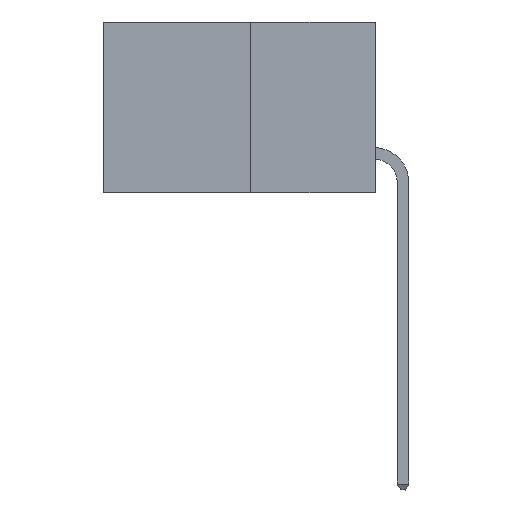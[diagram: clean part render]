
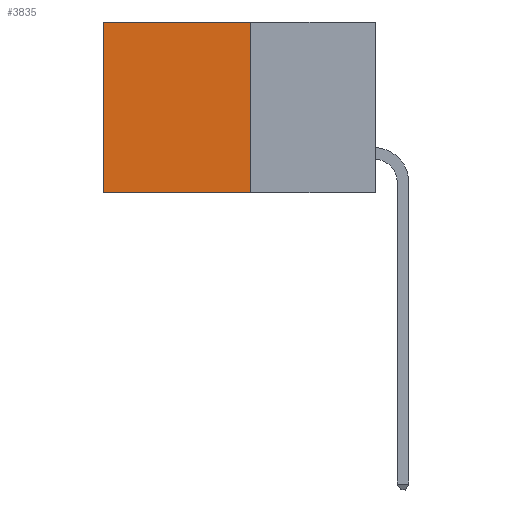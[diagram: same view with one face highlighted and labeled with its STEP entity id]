
A CAD part, left-side view. The second image highlights one B-rep face of the part: STEP entity #3835.
In plain terms, the highlighted planar face has unit normal (-1, 0, 0).
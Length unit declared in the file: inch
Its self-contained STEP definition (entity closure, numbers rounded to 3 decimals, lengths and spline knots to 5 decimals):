
#366 = FACE_OUTER_BOUND ( 'NONE', #6501, .T. ) ;
#469 = VECTOR ( 'NONE', #8511, 39.37008 ) ;
#616 = CARTESIAN_POINT ( 'NONE',  ( 0.277, 0.59, -0.37 ) ) ;
#716 = EDGE_CURVE ( 'NONE', #2247, #8234, #7925, .T. ) ;
#1585 = LINE ( 'NONE', #4110, #5914 ) ;
#1981 = DIRECTION ( 'NONE',  ( 0., 1., 0. ) ) ;
#2099 = CARTESIAN_POINT ( 'NONE',  ( 0.277, 0.27, 0. ) ) ;
#2247 = VERTEX_POINT ( 'NONE', #4051 ) ;
#2279 = LINE ( 'NONE', #2099, #9954 ) ;
#2424 = DIRECTION ( 'NONE',  ( 0., 0., -1. ) ) ;
#2600 = VERTEX_POINT ( 'NONE', #9516 ) ;
#3085 = LINE ( 'NONE', #8422, #469 ) ;
#3521 = ORIENTED_EDGE ( 'NONE', *, *, #5409, .T. ) ;
#3792 = DIRECTION ( 'NONE',  ( 1., 0., 0. ) ) ;
#3835 = ADVANCED_FACE ( 'NONE', ( #366 ), #4071, .F. ) ;
#3985 = AXIS2_PLACEMENT_3D ( 'NONE', #5148, #3792, #2424 ) ;
#4038 = DIRECTION ( 'NONE',  ( 0., 0., -1. ) ) ;
#4051 = CARTESIAN_POINT ( 'NONE',  ( 0.277, 0.27, -0.37 ) ) ;
#4071 = PLANE ( 'NONE',  #3985 ) ;
#4110 = CARTESIAN_POINT ( 'NONE',  ( 0.277, 0.27, -0.37 ) ) ;
#4239 = CARTESIAN_POINT ( 'NONE',  ( 0.277, 0.27, -0.37 ) ) ;
#4569 = CARTESIAN_POINT ( 'NONE',  ( 0.277, 0.27, 0. ) ) ;
#4856 = VERTEX_POINT ( 'NONE', #4569 ) ;
#5148 = CARTESIAN_POINT ( 'NONE',  ( 0.277, 0.27, -0.37 ) ) ;
#5409 = EDGE_CURVE ( 'NONE', #4856, #2600, #2279, .T. ) ;
#5639 = EDGE_CURVE ( 'NONE', #2600, #8234, #3085, .T. ) ;
#5822 = EDGE_CURVE ( 'NONE', #4856, #2247, #1585, .T. ) ;
#5914 = VECTOR ( 'NONE', #4038, 39.37008 ) ;
#6429 = ORIENTED_EDGE ( 'NONE', *, *, #5639, .T. ) ;
#6501 = EDGE_LOOP ( 'NONE', ( #6429, #8473, #9479, #3521 ) ) ;
#7109 = DIRECTION ( 'NONE',  ( 0., 1., 0. ) ) ;
#7925 = LINE ( 'NONE', #4239, #9641 ) ;
#8234 = VERTEX_POINT ( 'NONE', #616 ) ;
#8422 = CARTESIAN_POINT ( 'NONE',  ( 0.277, 0.59, -0.37 ) ) ;
#8473 = ORIENTED_EDGE ( 'NONE', *, *, #716, .F. ) ;
#8511 = DIRECTION ( 'NONE',  ( 0., 0., -1. ) ) ;
#9479 = ORIENTED_EDGE ( 'NONE', *, *, #5822, .F. ) ;
#9516 = CARTESIAN_POINT ( 'NONE',  ( 0.277, 0.59, 0. ) ) ;
#9641 = VECTOR ( 'NONE', #7109, 39.37008 ) ;
#9954 = VECTOR ( 'NONE', #1981, 39.37008 ) ;
